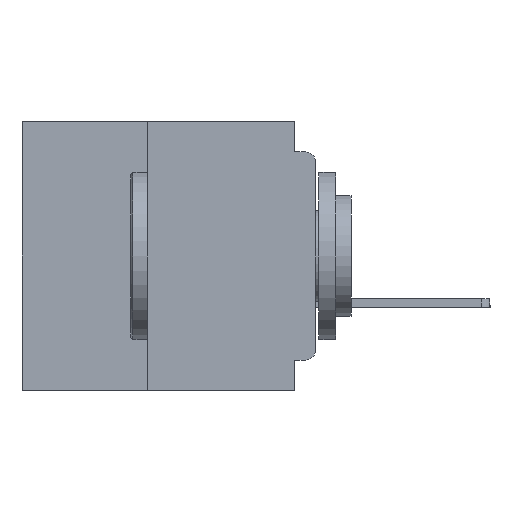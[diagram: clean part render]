
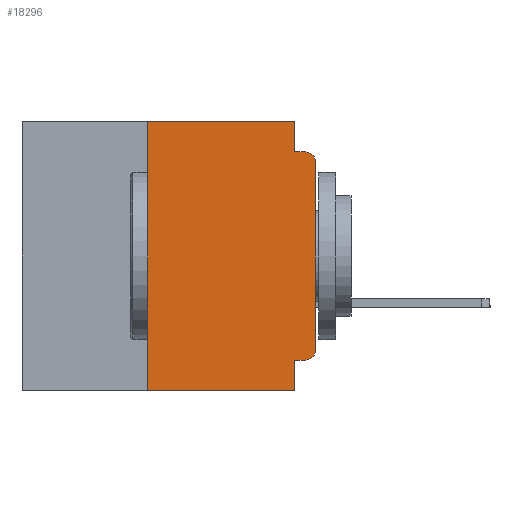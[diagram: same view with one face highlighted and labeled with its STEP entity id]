
A CAD part, left-side view. The second image highlights one B-rep face of the part: STEP entity #18296.
In plain terms, the highlighted planar face has unit normal (-1, 0, 0).
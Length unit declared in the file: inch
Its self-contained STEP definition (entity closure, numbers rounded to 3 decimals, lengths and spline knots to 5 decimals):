
#4463 = LINE ( 'NONE', #49198, #56267 ) ;
#5861 = FACE_OUTER_BOUND ( 'NONE', #58048, .T. ) ;
#6238 = CARTESIAN_POINT ( 'NONE',  ( 0., 0.031, -0.4 ) ) ;
#6363 = CARTESIAN_POINT ( 'NONE',  ( 0., 0., -0.06 ) ) ;
#7959 = DIRECTION ( 'NONE',  ( 0., -1., 0. ) ) ;
#8200 = AXIS2_PLACEMENT_3D ( 'NONE', #54566, #25562, #59390 ) ;
#8618 = CARTESIAN_POINT ( 'NONE',  ( 0., 0.437, -0.4 ) ) ;
#8699 = LINE ( 'NONE', #23463, #60366 ) ;
#9214 = DIRECTION ( 'NONE',  ( 0., 0., 1. ) ) ;
#10395 = LINE ( 'NONE', #56286, #46184 ) ;
#11951 = PLANE ( 'NONE',  #28490 ) ;
#12072 = VECTOR ( 'NONE', #9214, 39.37008 ) ;
#15129 = EDGE_CURVE ( 'NONE', #17598, #32430, #28537, .T. ) ;
#15164 = VECTOR ( 'NONE', #37820, 39.37008 ) ;
#16885 = DIRECTION ( 'NONE',  ( 1., 0., 0. ) ) ;
#17498 = EDGE_CURVE ( 'NONE', #23750, #17598, #4463, .T. ) ;
#17598 = VERTEX_POINT ( 'NONE', #6363 ) ;
#18296 = ADVANCED_FACE ( 'NONE', ( #5861 ), #11951, .F. ) ;
#21116 = VERTEX_POINT ( 'NONE', #56945 ) ;
#22390 = CARTESIAN_POINT ( 'NONE',  ( 0., 0.031, 0. ) ) ;
#23453 = EDGE_CURVE ( 'NONE', #29354, #32430, #46881, .T. ) ;
#23463 = CARTESIAN_POINT ( 'NONE',  ( 0., 0.437, 0. ) ) ;
#23750 = VERTEX_POINT ( 'NONE', #54664 ) ;
#23949 = VERTEX_POINT ( 'NONE', #22390 ) ;
#24087 = EDGE_CURVE ( 'NONE', #34668, #23949, #8699, .T. ) ;
#25137 = LINE ( 'NONE', #48160, #12072 ) ;
#25190 = ORIENTED_EDGE ( 'NONE', *, *, #15129, .T. ) ;
#25562 = DIRECTION ( 'NONE',  ( -1., 0., 0. ) ) ;
#26586 = CARTESIAN_POINT ( 'NONE',  ( 0., 0.031, -0.4 ) ) ;
#26725 = DIRECTION ( 'NONE',  ( -1., 0., 0. ) ) ;
#27386 = ORIENTED_EDGE ( 'NONE', *, *, #36749, .T. ) ;
#27746 = EDGE_CURVE ( 'NONE', #60773, #21116, #62129, .T. ) ;
#28435 = EDGE_CURVE ( 'NONE', #21116, #56738, #55277, .T. ) ;
#28490 = AXIS2_PLACEMENT_3D ( 'NONE', #41094, #16885, #50878 ) ;
#28537 = CIRCLE ( 'NONE', #8200, 0.015 ) ;
#29220 = ORIENTED_EDGE ( 'NONE', *, *, #27746, .F. ) ;
#29265 = CARTESIAN_POINT ( 'NONE',  ( 0., 0., -0.355 ) ) ;
#29354 = VERTEX_POINT ( 'NONE', #59566 ) ;
#32430 = VERTEX_POINT ( 'NONE', #37839 ) ;
#34118 = DIRECTION ( 'NONE',  ( 0., 1., 0. ) ) ;
#34571 = AXIS2_PLACEMENT_3D ( 'NONE', #55725, #26725, #60542 ) ;
#34668 = VERTEX_POINT ( 'NONE', #46269 ) ;
#34892 = VECTOR ( 'NONE', #34118, 39.37008 ) ;
#35707 = DIRECTION ( 'NONE',  ( 0., 0., -1. ) ) ;
#35871 = ORIENTED_EDGE ( 'NONE', *, *, #28435, .F. ) ;
#36749 = EDGE_CURVE ( 'NONE', #57712, #56738, #53971, .T. ) ;
#37820 = DIRECTION ( 'NONE',  ( 0., -1., 0. ) ) ;
#37839 = CARTESIAN_POINT ( 'NONE',  ( 0., 0.015, -0.045 ) ) ;
#38117 = EDGE_CURVE ( 'NONE', #23949, #29354, #10395, .T. ) ;
#39593 = ORIENTED_EDGE ( 'NONE', *, *, #17498, .T. ) ;
#40848 = ORIENTED_EDGE ( 'NONE', *, *, #42782, .F. ) ;
#41094 = CARTESIAN_POINT ( 'NONE',  ( 0., 0.437, 0. ) ) ;
#42025 = CARTESIAN_POINT ( 'NONE',  ( 0., 0., -0.045 ) ) ;
#42386 = VECTOR ( 'NONE', #35707, 39.37008 ) ;
#42782 = EDGE_CURVE ( 'NONE', #57712, #34668, #25137, .T. ) ;
#43370 = ORIENTED_EDGE ( 'NONE', *, *, #38117, .F. ) ;
#43395 = CIRCLE ( 'NONE', #34571, 0.015 ) ;
#46184 = VECTOR ( 'NONE', #61110, 39.37008 ) ;
#46269 = CARTESIAN_POINT ( 'NONE',  ( 0., 0.25, 0. ) ) ;
#46881 = LINE ( 'NONE', #42025, #58242 ) ;
#48160 = CARTESIAN_POINT ( 'NONE',  ( 0., 0.25, -0.4 ) ) ;
#48988 = DIRECTION ( 'NONE',  ( 0., 0., 1. ) ) ;
#49198 = CARTESIAN_POINT ( 'NONE',  ( 0., 0., 0. ) ) ;
#50878 = DIRECTION ( 'NONE',  ( 0., 0., -1. ) ) ;
#52696 = ORIENTED_EDGE ( 'NONE', *, *, #24087, .F. ) ;
#53971 = LINE ( 'NONE', #8618, #15164 ) ;
#54031 = ORIENTED_EDGE ( 'NONE', *, *, #23453, .F. ) ;
#54566 = CARTESIAN_POINT ( 'NONE',  ( 0., 0.015, -0.06 ) ) ;
#54664 = CARTESIAN_POINT ( 'NONE',  ( 0., 0., -0.34 ) ) ;
#55277 = LINE ( 'NONE', #6238, #42386 ) ;
#55725 = CARTESIAN_POINT ( 'NONE',  ( 0., 0.015, -0.34 ) ) ;
#56267 = VECTOR ( 'NONE', #48988, 39.37008 ) ;
#56286 = CARTESIAN_POINT ( 'NONE',  ( 0., 0.031, 0. ) ) ;
#56738 = VERTEX_POINT ( 'NONE', #26586 ) ;
#56945 = CARTESIAN_POINT ( 'NONE',  ( 0., 0.031, -0.355 ) ) ;
#57348 = EDGE_CURVE ( 'NONE', #60773, #23750, #43395, .T. ) ;
#57381 = DIRECTION ( 'NONE',  ( 0., -1., 0. ) ) ;
#57712 = VERTEX_POINT ( 'NONE', #58689 ) ;
#58048 = EDGE_LOOP ( 'NONE', ( #39593, #25190, #54031, #43370, #52696, #40848, #27386, #35871, #29220, #59656 ) ) ;
#58242 = VECTOR ( 'NONE', #7959, 39.37008 ) ;
#58689 = CARTESIAN_POINT ( 'NONE',  ( 0., 0.25, -0.4 ) ) ;
#59390 = DIRECTION ( 'NONE',  ( 0., 0., -1. ) ) ;
#59566 = CARTESIAN_POINT ( 'NONE',  ( 0., 0.031, -0.045 ) ) ;
#59656 = ORIENTED_EDGE ( 'NONE', *, *, #57348, .T. ) ;
#59673 = CARTESIAN_POINT ( 'NONE',  ( 0., 0.015, -0.355 ) ) ;
#60366 = VECTOR ( 'NONE', #57381, 39.37008 ) ;
#60542 = DIRECTION ( 'NONE',  ( 0., 0., -1. ) ) ;
#60773 = VERTEX_POINT ( 'NONE', #59673 ) ;
#61110 = DIRECTION ( 'NONE',  ( 0., 0., -1. ) ) ;
#62129 = LINE ( 'NONE', #29265, #34892 ) ;
